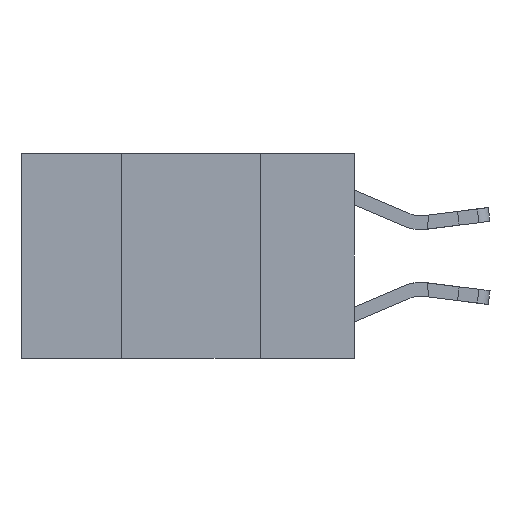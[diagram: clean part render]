
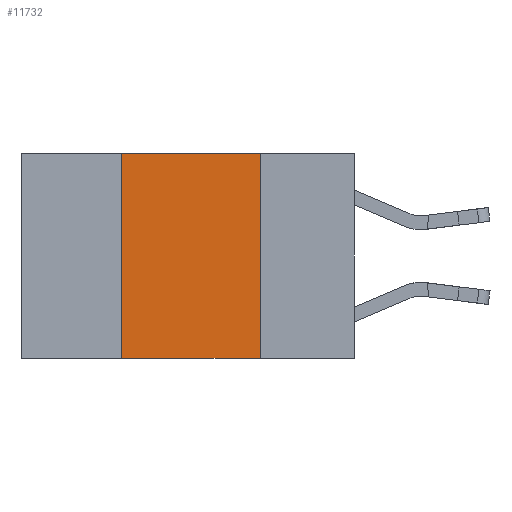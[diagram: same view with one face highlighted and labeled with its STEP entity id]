
A CAD part, left-side view. The second image highlights one B-rep face of the part: STEP entity #11732.
In plain terms, the highlighted planar face has unit normal (-1, 0, 0).
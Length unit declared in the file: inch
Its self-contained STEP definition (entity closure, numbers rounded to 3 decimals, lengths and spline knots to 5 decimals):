
#151 = DIRECTION ( 'NONE',  ( 0., -1., 0. ) ) ;
#515 = LINE ( 'NONE', #9276, #15188 ) ;
#587 = CARTESIAN_POINT ( 'NONE',  ( 0., 0.17, 0. ) ) ;
#1389 = VERTEX_POINT ( 'NONE', #4073 ) ;
#1393 = CARTESIAN_POINT ( 'NONE',  ( 0., 0.6, -0.37 ) ) ;
#1705 = DIRECTION ( 'NONE',  ( 1., 0., 0. ) ) ;
#1818 = VERTEX_POINT ( 'NONE', #9792 ) ;
#3266 = EDGE_CURVE ( 'NONE', #1389, #5715, #11930, .T. ) ;
#4073 = CARTESIAN_POINT ( 'NONE',  ( 0., 0.17, 0. ) ) ;
#4075 = CARTESIAN_POINT ( 'NONE',  ( 0., 0.42, 0. ) ) ;
#5715 = VERTEX_POINT ( 'NONE', #6527 ) ;
#5873 = VECTOR ( 'NONE', #12557, 39.37008 ) ;
#6096 = LINE ( 'NONE', #1393, #10850 ) ;
#6451 = ORIENTED_EDGE ( 'NONE', *, *, #3266, .F. ) ;
#6527 = CARTESIAN_POINT ( 'NONE',  ( 0., 0.17, -0.37 ) ) ;
#6641 = DIRECTION ( 'NONE',  ( 0., 0., -1. ) ) ;
#7230 = EDGE_LOOP ( 'NONE', ( #6451, #7555, #15833, #13004 ) ) ;
#7555 = ORIENTED_EDGE ( 'NONE', *, *, #11434, .F. ) ;
#7781 = PLANE ( 'NONE',  #14690 ) ;
#7969 = DIRECTION ( 'NONE',  ( 0., 0., -1. ) ) ;
#8989 = VECTOR ( 'NONE', #7969, 39.37008 ) ;
#9276 = CARTESIAN_POINT ( 'NONE',  ( 0., 0.6, 0. ) ) ;
#9791 = EDGE_CURVE ( 'NONE', #12421, #1818, #15379, .T. ) ;
#9792 = CARTESIAN_POINT ( 'NONE',  ( 0., 0.42, 0. ) ) ;
#10850 = VECTOR ( 'NONE', #151, 39.37008 ) ;
#11416 = FACE_OUTER_BOUND ( 'NONE', #7230, .T. ) ;
#11434 = EDGE_CURVE ( 'NONE', #1818, #1389, #515, .T. ) ;
#11732 = ADVANCED_FACE ( 'NONE', ( #11416 ), #7781, .F. ) ;
#11930 = LINE ( 'NONE', #587, #8989 ) ;
#12275 = CARTESIAN_POINT ( 'NONE',  ( 0., 0.42, -0.37 ) ) ;
#12421 = VERTEX_POINT ( 'NONE', #12275 ) ;
#12557 = DIRECTION ( 'NONE',  ( 0., 0., 1. ) ) ;
#13004 = ORIENTED_EDGE ( 'NONE', *, *, #13475, .T. ) ;
#13475 = EDGE_CURVE ( 'NONE', #12421, #5715, #6096, .T. ) ;
#13988 = CARTESIAN_POINT ( 'NONE',  ( 0., 0.6, 0. ) ) ;
#14104 = DIRECTION ( 'NONE',  ( 0., -1., 0. ) ) ;
#14690 = AXIS2_PLACEMENT_3D ( 'NONE', #13988, #1705, #6641 ) ;
#15188 = VECTOR ( 'NONE', #14104, 39.37008 ) ;
#15379 = LINE ( 'NONE', #4075, #5873 ) ;
#15833 = ORIENTED_EDGE ( 'NONE', *, *, #9791, .F. ) ;
